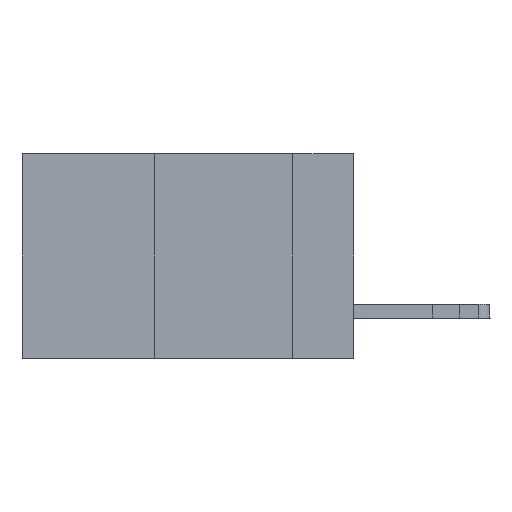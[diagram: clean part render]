
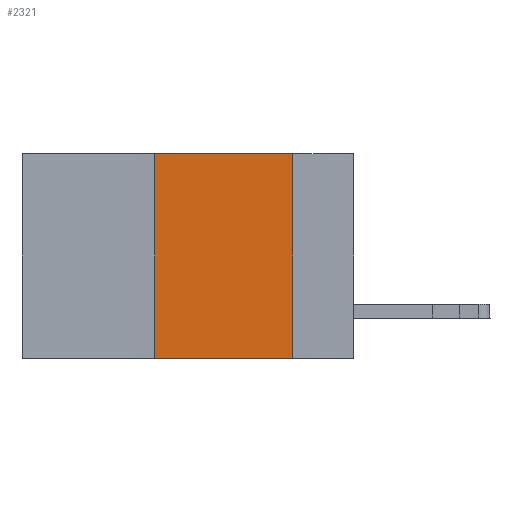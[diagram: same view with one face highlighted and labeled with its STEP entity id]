
A CAD part, left-side view. The second image highlights one B-rep face of the part: STEP entity #2321.
In plain terms, the highlighted planar face has unit normal (-1, 0, 0).
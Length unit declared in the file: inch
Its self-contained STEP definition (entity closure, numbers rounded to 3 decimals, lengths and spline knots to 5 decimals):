
#34 = CARTESIAN_POINT ( 'NONE',  ( 0., 0.6, -0.37 ) ) ;
#789 = EDGE_LOOP ( 'NONE', ( #5472, #16939, #6706, #7124 ) ) ;
#1704 = VERTEX_POINT ( 'NONE', #19811 ) ;
#1982 = VERTEX_POINT ( 'NONE', #6267 ) ;
#2185 = VERTEX_POINT ( 'NONE', #16967 ) ;
#2321 = ADVANCED_FACE ( 'NONE', ( #12445 ), #5738, .F. ) ;
#2979 = CARTESIAN_POINT ( 'NONE',  ( 0., 0.11, 0. ) ) ;
#2999 = LINE ( 'NONE', #15671, #14161 ) ;
#3051 = DIRECTION ( 'NONE',  ( 0., -1., 0. ) ) ;
#3206 = EDGE_CURVE ( 'NONE', #12186, #1704, #2999, .T. ) ;
#3468 = DIRECTION ( 'NONE',  ( 0., -1., 0. ) ) ;
#4872 = EDGE_CURVE ( 'NONE', #1982, #2185, #9608, .T. ) ;
#4918 = LINE ( 'NONE', #14056, #10519 ) ;
#5371 = CARTESIAN_POINT ( 'NONE',  ( 0., 0.36, -0.37 ) ) ;
#5472 = ORIENTED_EDGE ( 'NONE', *, *, #4872, .F. ) ;
#5680 = VECTOR ( 'NONE', #17214, 39.37008 ) ;
#5738 = PLANE ( 'NONE',  #6259 ) ;
#6259 = AXIS2_PLACEMENT_3D ( 'NONE', #9265, #12348, #18739 ) ;
#6267 = CARTESIAN_POINT ( 'NONE',  ( 0., 0.11, 0. ) ) ;
#6706 = ORIENTED_EDGE ( 'NONE', *, *, #3206, .F. ) ;
#7124 = ORIENTED_EDGE ( 'NONE', *, *, #18465, .T. ) ;
#7647 = EDGE_CURVE ( 'NONE', #1704, #1982, #4918, .T. ) ;
#9265 = CARTESIAN_POINT ( 'NONE',  ( 0., 0.6, 0. ) ) ;
#9608 = LINE ( 'NONE', #2979, #5680 ) ;
#10519 = VECTOR ( 'NONE', #3051, 39.37008 ) ;
#12186 = VERTEX_POINT ( 'NONE', #5371 ) ;
#12348 = DIRECTION ( 'NONE',  ( 1., 0., 0. ) ) ;
#12445 = FACE_OUTER_BOUND ( 'NONE', #789, .T. ) ;
#13376 = VECTOR ( 'NONE', #3468, 39.37008 ) ;
#14002 = DIRECTION ( 'NONE',  ( 0., 0., 1. ) ) ;
#14056 = CARTESIAN_POINT ( 'NONE',  ( 0., 0.6, 0. ) ) ;
#14161 = VECTOR ( 'NONE', #14002, 39.37008 ) ;
#15671 = CARTESIAN_POINT ( 'NONE',  ( 0., 0.36, 0. ) ) ;
#16939 = ORIENTED_EDGE ( 'NONE', *, *, #7647, .F. ) ;
#16967 = CARTESIAN_POINT ( 'NONE',  ( 0., 0.11, -0.37 ) ) ;
#17214 = DIRECTION ( 'NONE',  ( 0., 0., -1. ) ) ;
#17711 = LINE ( 'NONE', #34, #13376 ) ;
#18465 = EDGE_CURVE ( 'NONE', #12186, #2185, #17711, .T. ) ;
#18739 = DIRECTION ( 'NONE',  ( 0., 0., -1. ) ) ;
#19811 = CARTESIAN_POINT ( 'NONE',  ( 0., 0.36, 0. ) ) ;
